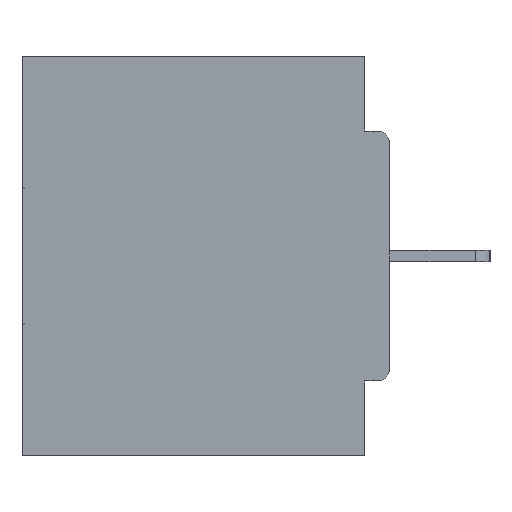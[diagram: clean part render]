
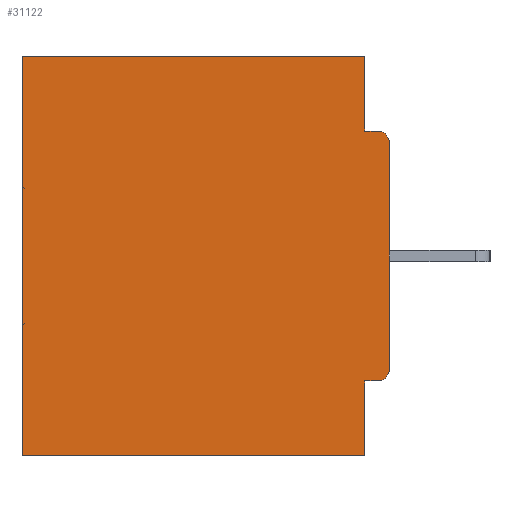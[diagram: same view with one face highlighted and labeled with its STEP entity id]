
A CAD part, left-side view. The second image highlights one B-rep face of the part: STEP entity #31122.
In plain terms, the highlighted planar face has unit normal (-1, 0, 0).
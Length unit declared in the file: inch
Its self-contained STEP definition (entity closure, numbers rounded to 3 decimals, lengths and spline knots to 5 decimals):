
#61 = CARTESIAN_POINT ( 'NONE',  ( 0.298, 0.46, 0. ) ) ;
#985 = DIRECTION ( 'NONE',  ( 0., -1., 0. ) ) ;
#1372 = EDGE_CURVE ( 'NONE', #23314, #12013, #4745, .T. ) ;
#1427 = VECTOR ( 'NONE', #16938, 39.37008 ) ;
#2023 = CARTESIAN_POINT ( 'NONE',  ( 0.298, 0.031, -0.0935 ) ) ;
#2243 = VERTEX_POINT ( 'NONE', #33435 ) ;
#2867 = DIRECTION ( 'NONE',  ( 0., 0., -1. ) ) ;
#2930 = CARTESIAN_POINT ( 'NONE',  ( 0.298, 0.015, -0.4065 ) ) ;
#3143 = DIRECTION ( 'NONE',  ( 0., 1., 0. ) ) ;
#3237 = CARTESIAN_POINT ( 'NONE',  ( 0.298, 0., 0. ) ) ;
#3774 = LINE ( 'NONE', #61, #17831 ) ;
#4511 = CARTESIAN_POINT ( 'NONE',  ( 0.298, 0.015, -0.3915 ) ) ;
#4575 = ORIENTED_EDGE ( 'NONE', *, *, #35441, .T. ) ;
#4745 = LINE ( 'NONE', #17393, #35518 ) ;
#4768 = DIRECTION ( 'NONE',  ( -1., 0., 0. ) ) ;
#5648 = CARTESIAN_POINT ( 'NONE',  ( 0.298, 0.015, -0.1085 ) ) ;
#5893 = DIRECTION ( 'NONE',  ( 0., 0., -1. ) ) ;
#6608 = ORIENTED_EDGE ( 'NONE', *, *, #32346, .F. ) ;
#6866 = CARTESIAN_POINT ( 'NONE',  ( 0.298, 0.015, -0.0935 ) ) ;
#7754 = FACE_OUTER_BOUND ( 'NONE', #10743, .T. ) ;
#7883 = DIRECTION ( 'NONE',  ( 0., 1., 0. ) ) ;
#8311 = CIRCLE ( 'NONE', #24959, 0.015 ) ;
#8751 = DIRECTION ( 'NONE',  ( 0., 0., -1. ) ) ;
#9294 = DIRECTION ( 'NONE',  ( 0., 0., -1. ) ) ;
#9409 = CARTESIAN_POINT ( 'NONE',  ( 0.298, 0., -0.0935 ) ) ;
#10743 = EDGE_LOOP ( 'NONE', ( #22461, #13043, #29192, #24651, #23993, #23498, #14929, #26391, #4575, #6608 ) ) ;
#10759 = EDGE_CURVE ( 'NONE', #28894, #34822, #28700, .T. ) ;
#10947 = LINE ( 'NONE', #18914, #20183 ) ;
#11191 = VERTEX_POINT ( 'NONE', #2023 ) ;
#11917 = CARTESIAN_POINT ( 'NONE',  ( 0.298, 0.031, -0.4065 ) ) ;
#12013 = VERTEX_POINT ( 'NONE', #15019 ) ;
#12145 = CARTESIAN_POINT ( 'NONE',  ( 0.298, 0., -0.1085 ) ) ;
#12604 = EDGE_CURVE ( 'NONE', #2243, #24703, #10947, .T. ) ;
#13043 = ORIENTED_EDGE ( 'NONE', *, *, #34483, .F. ) ;
#14238 = PLANE ( 'NONE',  #30495 ) ;
#14929 = ORIENTED_EDGE ( 'NONE', *, *, #27432, .F. ) ;
#15019 = CARTESIAN_POINT ( 'NONE',  ( 0.298, 0.46, -0.5 ) ) ;
#16938 = DIRECTION ( 'NONE',  ( 0., 1., 0. ) ) ;
#17393 = CARTESIAN_POINT ( 'NONE',  ( 0.298, 0., -0.5 ) ) ;
#17831 = VECTOR ( 'NONE', #33512, 39.37008 ) ;
#18457 = VERTEX_POINT ( 'NONE', #23351 ) ;
#18846 = VECTOR ( 'NONE', #985, 39.37008 ) ;
#18914 = CARTESIAN_POINT ( 'NONE',  ( 0.298, 0., 0. ) ) ;
#19883 = CARTESIAN_POINT ( 'NONE',  ( 0.298, 0., -0.4065 ) ) ;
#20135 = EDGE_CURVE ( 'NONE', #24703, #12013, #3774, .T. ) ;
#20183 = VECTOR ( 'NONE', #7883, 39.37008 ) ;
#21747 = LINE ( 'NONE', #3237, #30108 ) ;
#22461 = ORIENTED_EDGE ( 'NONE', *, *, #35466, .T. ) ;
#22675 = VECTOR ( 'NONE', #9294, 39.37008 ) ;
#23314 = VERTEX_POINT ( 'NONE', #24399 ) ;
#23351 = CARTESIAN_POINT ( 'NONE',  ( 0.298, 0., -0.3915 ) ) ;
#23498 = ORIENTED_EDGE ( 'NONE', *, *, #1372, .F. ) ;
#23607 = LINE ( 'NONE', #26039, #33702 ) ;
#23993 = ORIENTED_EDGE ( 'NONE', *, *, #20135, .T. ) ;
#24178 = DIRECTION ( 'NONE',  ( 0., 0., -1. ) ) ;
#24375 = VERTEX_POINT ( 'NONE', #12145 ) ;
#24399 = CARTESIAN_POINT ( 'NONE',  ( 0.298, 0.031, -0.5 ) ) ;
#24412 = LINE ( 'NONE', #29174, #22675 ) ;
#24651 = ORIENTED_EDGE ( 'NONE', *, *, #12604, .T. ) ;
#24703 = VERTEX_POINT ( 'NONE', #35272 ) ;
#24959 = AXIS2_PLACEMENT_3D ( 'NONE', #5648, #31193, #5893 ) ;
#25419 = CIRCLE ( 'NONE', #35050, 0.015 ) ;
#25529 = CARTESIAN_POINT ( 'NONE',  ( 0.298, 0., 0. ) ) ;
#26039 = CARTESIAN_POINT ( 'NONE',  ( 0.298, 0.031, -0.5 ) ) ;
#26334 = LINE ( 'NONE', #9409, #18846 ) ;
#26391 = ORIENTED_EDGE ( 'NONE', *, *, #10759, .F. ) ;
#27432 = EDGE_CURVE ( 'NONE', #34822, #23314, #23607, .T. ) ;
#28351 = DIRECTION ( 'NONE',  ( 1., 0., 0. ) ) ;
#28700 = LINE ( 'NONE', #19883, #1427 ) ;
#28894 = VERTEX_POINT ( 'NONE', #2930 ) ;
#29174 = CARTESIAN_POINT ( 'NONE',  ( 0.298, 0.031, -0.5 ) ) ;
#29192 = ORIENTED_EDGE ( 'NONE', *, *, #29293, .F. ) ;
#29293 = EDGE_CURVE ( 'NONE', #2243, #11191, #24412, .T. ) ;
#30108 = VECTOR ( 'NONE', #2867, 39.37008 ) ;
#30495 = AXIS2_PLACEMENT_3D ( 'NONE', #25529, #28351, #30823 ) ;
#30823 = DIRECTION ( 'NONE',  ( 0., 0., -1. ) ) ;
#31122 = ADVANCED_FACE ( 'NONE', ( #7754 ), #14238, .F. ) ;
#31193 = DIRECTION ( 'NONE',  ( -1., 0., 0. ) ) ;
#32346 = EDGE_CURVE ( 'NONE', #24375, #18457, #21747, .T. ) ;
#33435 = CARTESIAN_POINT ( 'NONE',  ( 0.298, 0.031, 0. ) ) ;
#33512 = DIRECTION ( 'NONE',  ( 0., 0., -1. ) ) ;
#33702 = VECTOR ( 'NONE', #8751, 39.37008 ) ;
#34483 = EDGE_CURVE ( 'NONE', #11191, #35639, #26334, .T. ) ;
#34822 = VERTEX_POINT ( 'NONE', #11917 ) ;
#35050 = AXIS2_PLACEMENT_3D ( 'NONE', #4511, #4768, #24178 ) ;
#35272 = CARTESIAN_POINT ( 'NONE',  ( 0.298, 0.46, 0. ) ) ;
#35441 = EDGE_CURVE ( 'NONE', #28894, #18457, #25419, .T. ) ;
#35466 = EDGE_CURVE ( 'NONE', #24375, #35639, #8311, .T. ) ;
#35518 = VECTOR ( 'NONE', #3143, 39.37008 ) ;
#35639 = VERTEX_POINT ( 'NONE', #6866 ) ;
